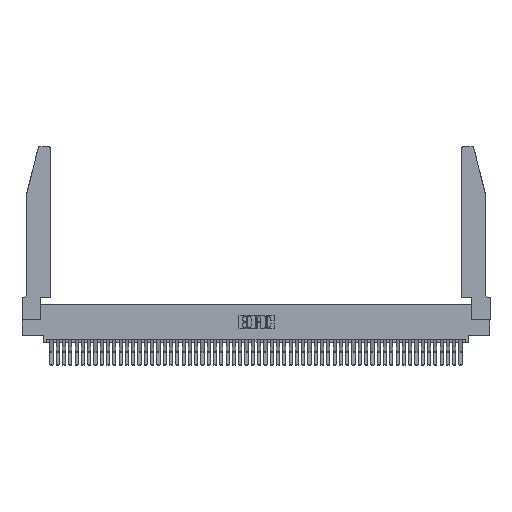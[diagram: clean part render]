
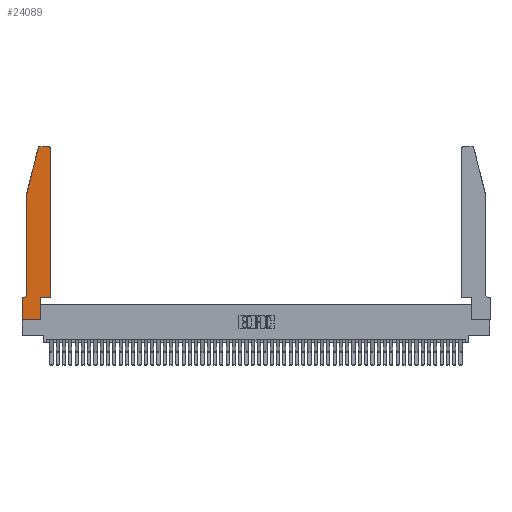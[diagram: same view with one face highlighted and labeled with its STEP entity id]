
A CAD part, top view. The second image highlights one B-rep face of the part: STEP entity #24089.
In plain terms, the highlighted planar face has unit normal (0, 0, 1).
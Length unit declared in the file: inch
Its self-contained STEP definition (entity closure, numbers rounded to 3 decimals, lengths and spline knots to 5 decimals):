
#286 = EDGE_CURVE ( 'NONE', #26110, #41033, #2419, .T. ) ;
#289 = CARTESIAN_POINT ( 'NONE',  ( 0.284, 2.72, 0.37 ) ) ;
#1085 = VECTOR ( 'NONE', #24165, 39.37008 ) ;
#1100 = ORIENTED_EDGE ( 'NONE', *, *, #47666, .T. ) ;
#2400 = CARTESIAN_POINT ( 'NONE',  ( 0.4505, 2.72, 0.37 ) ) ;
#2419 = LINE ( 'NONE', #44671, #1085 ) ;
#2982 = CARTESIAN_POINT ( 'NONE',  ( 0.4505, 0.35, 0.37 ) ) ;
#3444 = DIRECTION ( 'NONE',  ( 0., 1., 0. ) ) ;
#3822 = VECTOR ( 'NONE', #37783, 39.37008 ) ;
#4057 = CARTESIAN_POINT ( 'NONE',  ( 0.0055, 0.35, 0.37 ) ) ;
#4130 = ORIENTED_EDGE ( 'NONE', *, *, #51106, .T. ) ;
#4139 = VECTOR ( 'NONE', #22343, 39.37008 ) ;
#4525 = DIRECTION ( 'NONE',  ( 1., 0., 0. ) ) ;
#4624 = AXIS2_PLACEMENT_3D ( 'NONE', #44621, #19945, #48701 ) ;
#5358 = ORIENTED_EDGE ( 'NONE', *, *, #43531, .T. ) ;
#5621 = EDGE_CURVE ( 'NONE', #45546, #45051, #36927, .T. ) ;
#6157 = CARTESIAN_POINT ( 'NONE',  ( 0.0755, 0.42, 0.37 ) ) ;
#6963 = ORIENTED_EDGE ( 'NONE', *, *, #286, .T. ) ;
#7091 = CARTESIAN_POINT ( 'NONE',  ( 0.2605, 2.75, 0.37 ) ) ;
#7172 = DIRECTION ( 'NONE',  ( 1., 0., 0. ) ) ;
#8439 = EDGE_CURVE ( 'NONE', #45051, #31481, #18186, .T. ) ;
#8476 = EDGE_CURVE ( 'NONE', #31481, #34506, #25301, .T. ) ;
#8998 = EDGE_CURVE ( 'NONE', #41033, #49439, #12935, .T. ) ;
#9329 = EDGE_CURVE ( 'NONE', #16456, #26110, #49596, .T. ) ;
#9658 = CARTESIAN_POINT ( 'NONE',  ( 0.2865, 0., 0.37 ) ) ;
#10065 = VECTOR ( 'NONE', #24253, 39.37008 ) ;
#10556 = VERTEX_POINT ( 'NONE', #40837 ) ;
#11340 = DIRECTION ( 'NONE',  ( -1., 0., 0. ) ) ;
#11604 = PLANE ( 'NONE',  #4624 ) ;
#12641 = CARTESIAN_POINT ( 'NONE',  ( 0.0755, 2., 0.37 ) ) ;
#12935 = CIRCLE ( 'NONE', #48216, 0.07 ) ;
#14143 = CARTESIAN_POINT ( 'NONE',  ( 0., 0., 0.37 ) ) ;
#16102 = AXIS2_PLACEMENT_3D ( 'NONE', #19318, #48109, #23523 ) ;
#16456 = VERTEX_POINT ( 'NONE', #37060 ) ;
#16793 = DIRECTION ( 'NONE',  ( -0.239, -0.971, 0. ) ) ;
#17216 = CIRCLE ( 'NONE', #49502, 0.03 ) ;
#18186 = CIRCLE ( 'NONE', #16102, 0.03 ) ;
#18951 = LINE ( 'NONE', #44728, #27376 ) ;
#19318 = CARTESIAN_POINT ( 'NONE',  ( 0.4205, 2.72, 0.37 ) ) ;
#19429 = ORIENTED_EDGE ( 'NONE', *, *, #31892, .T. ) ;
#19945 = DIRECTION ( 'NONE',  ( 0., 0., 1. ) ) ;
#20085 = CARTESIAN_POINT ( 'NONE',  ( 0., 0., 0.37 ) ) ;
#20314 = ORIENTED_EDGE ( 'NONE', *, *, #42598, .T. ) ;
#21454 = ORIENTED_EDGE ( 'NONE', *, *, #8439, .T. ) ;
#21901 = LINE ( 'NONE', #2982, #52044 ) ;
#22343 = DIRECTION ( 'NONE',  ( 0., -1., 0. ) ) ;
#22508 = VERTEX_POINT ( 'NONE', #31771 ) ;
#22681 = CARTESIAN_POINT ( 'NONE',  ( 0.0055, 0.42, 0.37 ) ) ;
#23523 = DIRECTION ( 'NONE',  ( 1., 0., 0. ) ) ;
#23625 = ORIENTED_EDGE ( 'NONE', *, *, #5621, .T. ) ;
#24024 = VECTOR ( 'NONE', #11340, 39.37008 ) ;
#24089 = ADVANCED_FACE ( 'NONE', ( #33446 ), #11604, .T. ) ;
#24165 = DIRECTION ( 'NONE',  ( 0., -1., 0. ) ) ;
#24253 = DIRECTION ( 'NONE',  ( 1., 0., 0. ) ) ;
#24508 = ORIENTED_EDGE ( 'NONE', *, *, #9329, .T. ) ;
#24690 = EDGE_CURVE ( 'NONE', #35435, #48564, #48763, .T. ) ;
#25227 = CARTESIAN_POINT ( 'NONE',  ( 0., 0., 0.37 ) ) ;
#25301 = LINE ( 'NONE', #7091, #24024 ) ;
#25603 = CARTESIAN_POINT ( 'NONE',  ( 0.4205, 2.75, 0.37 ) ) ;
#26110 = VERTEX_POINT ( 'NONE', #46403 ) ;
#26164 = ORIENTED_EDGE ( 'NONE', *, *, #8476, .T. ) ;
#26829 = DIRECTION ( 'NONE',  ( -1., 0., 0. ) ) ;
#27376 = VECTOR ( 'NONE', #3444, 39.37008 ) ;
#27801 = VECTOR ( 'NONE', #16793, 39.37008 ) ;
#29435 = DIRECTION ( 'NONE',  ( 0., 0., 1. ) ) ;
#31481 = VERTEX_POINT ( 'NONE', #25603 ) ;
#31771 = CARTESIAN_POINT ( 'NONE',  ( 0.2865, 0.35, 0.37 ) ) ;
#31892 = EDGE_CURVE ( 'NONE', #22508, #45546, #21901, .T. ) ;
#31987 = DIRECTION ( 'NONE',  ( -1., 0., 0. ) ) ;
#33446 = FACE_OUTER_BOUND ( 'NONE', #50720, .T. ) ;
#33650 = CARTESIAN_POINT ( 'NONE',  ( 0.4505, 0.35, 0.37 ) ) ;
#34506 = VERTEX_POINT ( 'NONE', #44392 ) ;
#34800 = VECTOR ( 'NONE', #31987, 39.37008 ) ;
#35435 = VERTEX_POINT ( 'NONE', #25227 ) ;
#36082 = LINE ( 'NONE', #52338, #34800 ) ;
#36927 = LINE ( 'NONE', #33650, #3822 ) ;
#37060 = CARTESIAN_POINT ( 'NONE',  ( 0.25487, 2.72718, 0.37 ) ) ;
#37246 = LINE ( 'NONE', #14143, #4139 ) ;
#37783 = DIRECTION ( 'NONE',  ( 0., 1., 0. ) ) ;
#38646 = CARTESIAN_POINT ( 'NONE',  ( 0.4505, 0.35, 0.37 ) ) ;
#38929 = ORIENTED_EDGE ( 'NONE', *, *, #8998, .T. ) ;
#40837 = CARTESIAN_POINT ( 'NONE',  ( 0., 0.35, 0.37 ) ) ;
#41033 = VERTEX_POINT ( 'NONE', #6157 ) ;
#41064 = ORIENTED_EDGE ( 'NONE', *, *, #24690, .T. ) ;
#42598 = EDGE_CURVE ( 'NONE', #10556, #35435, #37246, .T. ) ;
#43531 = EDGE_CURVE ( 'NONE', #34506, #16456, #17216, .T. ) ;
#44392 = CARTESIAN_POINT ( 'NONE',  ( 0.284, 2.75, 0.37 ) ) ;
#44621 = CARTESIAN_POINT ( 'NONE',  ( 0., 0.35, 0.37 ) ) ;
#44671 = CARTESIAN_POINT ( 'NONE',  ( 0.0755, 2., 0.37 ) ) ;
#44728 = CARTESIAN_POINT ( 'NONE',  ( 0.2865, 0.35, 0.37 ) ) ;
#45051 = VERTEX_POINT ( 'NONE', #2400 ) ;
#45546 = VERTEX_POINT ( 'NONE', #38646 ) ;
#46403 = CARTESIAN_POINT ( 'NONE',  ( 0.0755, 2., 0.37 ) ) ;
#47666 = EDGE_CURVE ( 'NONE', #48564, #22508, #18951, .T. ) ;
#48109 = DIRECTION ( 'NONE',  ( 0., 0., 1. ) ) ;
#48216 = AXIS2_PLACEMENT_3D ( 'NONE', #22681, #51344, #26829 ) ;
#48564 = VERTEX_POINT ( 'NONE', #9658 ) ;
#48701 = DIRECTION ( 'NONE',  ( 1., 0., 0. ) ) ;
#48763 = LINE ( 'NONE', #20085, #10065 ) ;
#49439 = VERTEX_POINT ( 'NONE', #4057 ) ;
#49502 = AXIS2_PLACEMENT_3D ( 'NONE', #289, #29435, #4525 ) ;
#49596 = LINE ( 'NONE', #12641, #27801 ) ;
#50720 = EDGE_LOOP ( 'NONE', ( #26164, #5358, #24508, #6963, #38929, #4130, #20314, #41064, #1100, #19429, #23625, #21454 ) ) ;
#51106 = EDGE_CURVE ( 'NONE', #49439, #10556, #36082, .T. ) ;
#51344 = DIRECTION ( 'NONE',  ( 0., 0., -1. ) ) ;
#52044 = VECTOR ( 'NONE', #7172, 39.37008 ) ;
#52338 = CARTESIAN_POINT ( 'NONE',  ( 0.0755, 0.35, 0.37 ) ) ;
